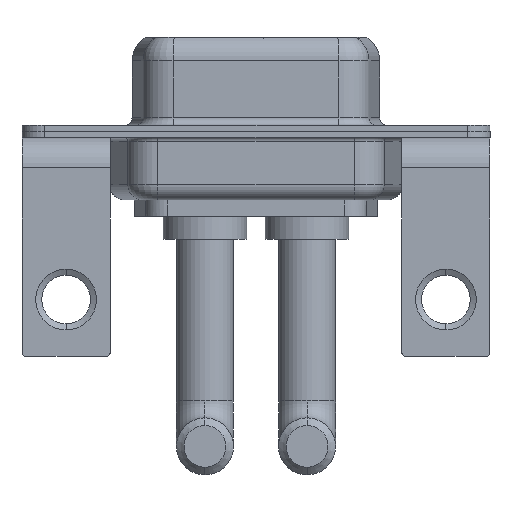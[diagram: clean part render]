
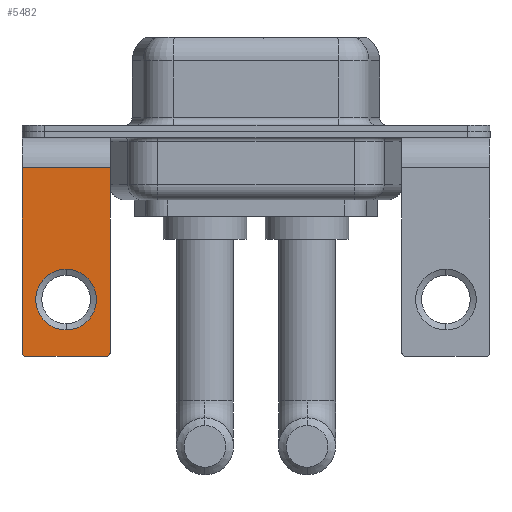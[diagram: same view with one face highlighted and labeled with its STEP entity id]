
A CAD part, front view. The second image highlights one B-rep face of the part: STEP entity #5482.
In plain terms, the highlighted planar face has unit normal (0, -1, 0).
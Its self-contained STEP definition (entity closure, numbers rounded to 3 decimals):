
#71 = VERTEX_POINT ( 'NONE', #4264 ) ;
#89 = FACE_BOUND ( 'NONE', #2845, .T. ) ;
#117 = EDGE_CURVE ( 'NONE', #13231, #1016, #8949, .T. ) ;
#566 = LINE ( 'NONE', #4906, #10366 ) ;
#873 = DIRECTION ( 'NONE',  ( 0., -1., 0. ) ) ;
#969 = CARTESIAN_POINT ( 'NONE',  ( 0., -6.25, -13.07 ) ) ;
#1016 = VERTEX_POINT ( 'NONE', #969 ) ;
#1435 = AXIS2_PLACEMENT_3D ( 'NONE', #4193, #9534, #3176 ) ;
#1779 = CIRCLE ( 'NONE', #6809, 2. ) ;
#1868 = CARTESIAN_POINT ( 'NONE',  ( 2.65, -6.25, -14.8 ) ) ;
#2089 = CIRCLE ( 'NONE', #13711, 0.25 ) ;
#2404 = FACE_OUTER_BOUND ( 'NONE', #8556, .T. ) ;
#2618 = DIRECTION ( 'NONE',  ( 0., 0., -1. ) ) ;
#2708 = VERTEX_POINT ( 'NONE', #12235 ) ;
#2845 = EDGE_LOOP ( 'NONE', ( #10508, #7983 ) ) ;
#3139 = VERTEX_POINT ( 'NONE', #13947 ) ;
#3176 = DIRECTION ( 'NONE',  ( 0., 0., 1. ) ) ;
#3445 = CARTESIAN_POINT ( 'NONE',  ( 2.9, -6.25, -2.4 ) ) ;
#3611 = LINE ( 'NONE', #13611, #5722 ) ;
#3709 = CARTESIAN_POINT ( 'NONE',  ( 2.9, -6.25, -2.4 ) ) ;
#3814 = DIRECTION ( 'NONE',  ( -1., 0., 0. ) ) ;
#3901 = CARTESIAN_POINT ( 'NONE',  ( 2.9, -6.25, -14.8 ) ) ;
#3912 = DIRECTION ( 'NONE',  ( 0., 1., 0. ) ) ;
#4056 = AXIS2_PLACEMENT_3D ( 'NONE', #13122, #8765, #6772 ) ;
#4178 = ORIENTED_EDGE ( 'NONE', *, *, #13459, .T. ) ;
#4193 = CARTESIAN_POINT ( 'NONE',  ( 0., -6.25, -11.07 ) ) ;
#4264 = CARTESIAN_POINT ( 'NONE',  ( -2.9, -6.25, -2.4 ) ) ;
#4570 = DIRECTION ( 'NONE',  ( 0., 0., 1. ) ) ;
#4602 = ORIENTED_EDGE ( 'NONE', *, *, #6999, .T. ) ;
#4816 = VERTEX_POINT ( 'NONE', #1868 ) ;
#4906 = CARTESIAN_POINT ( 'NONE',  ( 2.9, -6.25, -2.4 ) ) ;
#5211 = EDGE_CURVE ( 'NONE', #1016, #13231, #1779, .T. ) ;
#5482 = ADVANCED_FACE ( 'NONE', ( #89, #2404 ), #5707, .F. ) ;
#5707 = PLANE ( 'NONE',  #4056 ) ;
#5722 = VECTOR ( 'NONE', #2618, 1000. ) ;
#5734 = VECTOR ( 'NONE', #12300, 1000. ) ;
#5938 = AXIS2_PLACEMENT_3D ( 'NONE', #9679, #873, #7399 ) ;
#6146 = LINE ( 'NONE', #3901, #13723 ) ;
#6174 = CIRCLE ( 'NONE', #5938, 0.25 ) ;
#6569 = VERTEX_POINT ( 'NONE', #13143 ) ;
#6772 = DIRECTION ( 'NONE',  ( 0., 0., 1. ) ) ;
#6809 = AXIS2_PLACEMENT_3D ( 'NONE', #9341, #3912, #10263 ) ;
#6999 = EDGE_CURVE ( 'NONE', #3139, #6569, #6174, .T. ) ;
#7003 = CARTESIAN_POINT ( 'NONE',  ( 0., -6.25, -9.07 ) ) ;
#7051 = ORIENTED_EDGE ( 'NONE', *, *, #12752, .F. ) ;
#7399 = DIRECTION ( 'NONE',  ( 0., 0., 1. ) ) ;
#7755 = DIRECTION ( 'NONE',  ( 0., -1., 0. ) ) ;
#7935 = LINE ( 'NONE', #3445, #5734 ) ;
#7983 = ORIENTED_EDGE ( 'NONE', *, *, #117, .T. ) ;
#8102 = ORIENTED_EDGE ( 'NONE', *, *, #10423, .T. ) ;
#8556 = EDGE_LOOP ( 'NONE', ( #12655, #4602, #11120, #4178, #7051, #8102 ) ) ;
#8765 = DIRECTION ( 'NONE',  ( 0., 1., 0. ) ) ;
#8949 = CIRCLE ( 'NONE', #1435, 2. ) ;
#9098 = EDGE_CURVE ( 'NONE', #4816, #6569, #6146, .T. ) ;
#9341 = CARTESIAN_POINT ( 'NONE',  ( 0., -6.25, -11.07 ) ) ;
#9534 = DIRECTION ( 'NONE',  ( 0., 1., 0. ) ) ;
#9679 = CARTESIAN_POINT ( 'NONE',  ( -2.65, -6.25, -14.55 ) ) ;
#9906 = CARTESIAN_POINT ( 'NONE',  ( 2.65, -6.25, -14.55 ) ) ;
#10263 = DIRECTION ( 'NONE',  ( 0., 0., 1. ) ) ;
#10366 = VECTOR ( 'NONE', #3814, 1000. ) ;
#10423 = EDGE_CURVE ( 'NONE', #13270, #71, #566, .T. ) ;
#10462 = DIRECTION ( 'NONE',  ( -1., 0., 0. ) ) ;
#10508 = ORIENTED_EDGE ( 'NONE', *, *, #5211, .T. ) ;
#11120 = ORIENTED_EDGE ( 'NONE', *, *, #9098, .F. ) ;
#11888 = EDGE_CURVE ( 'NONE', #71, #3139, #3611, .T. ) ;
#12235 = CARTESIAN_POINT ( 'NONE',  ( 2.9, -6.25, -14.55 ) ) ;
#12300 = DIRECTION ( 'NONE',  ( 0., 0., -1. ) ) ;
#12655 = ORIENTED_EDGE ( 'NONE', *, *, #11888, .T. ) ;
#12752 = EDGE_CURVE ( 'NONE', #13270, #2708, #7935, .T. ) ;
#13122 = CARTESIAN_POINT ( 'NONE',  ( 2.9, -6.25, -2.4 ) ) ;
#13143 = CARTESIAN_POINT ( 'NONE',  ( -2.65, -6.25, -14.8 ) ) ;
#13231 = VERTEX_POINT ( 'NONE', #7003 ) ;
#13270 = VERTEX_POINT ( 'NONE', #3709 ) ;
#13459 = EDGE_CURVE ( 'NONE', #4816, #2708, #2089, .T. ) ;
#13611 = CARTESIAN_POINT ( 'NONE',  ( -2.9, -6.25, -2.4 ) ) ;
#13711 = AXIS2_PLACEMENT_3D ( 'NONE', #9906, #7755, #4570 ) ;
#13723 = VECTOR ( 'NONE', #10462, 1000. ) ;
#13947 = CARTESIAN_POINT ( 'NONE',  ( -2.9, -6.25, -14.55 ) ) ;
